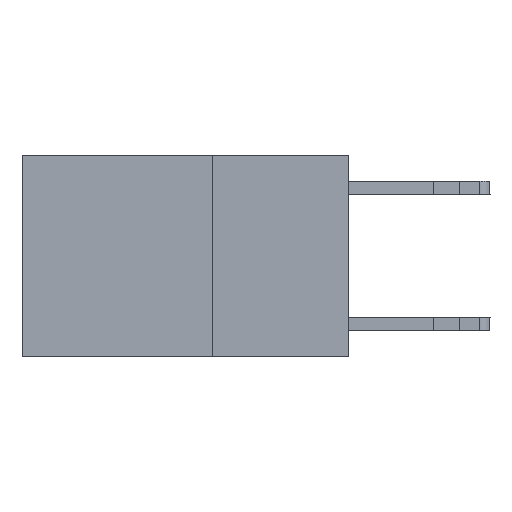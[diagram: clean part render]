
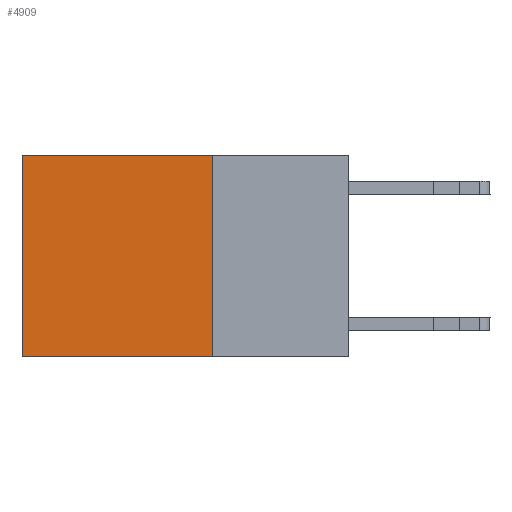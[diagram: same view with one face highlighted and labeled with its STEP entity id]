
A CAD part, left-side view. The second image highlights one B-rep face of the part: STEP entity #4909.
In plain terms, the highlighted planar face has unit normal (-1, 0, 0).
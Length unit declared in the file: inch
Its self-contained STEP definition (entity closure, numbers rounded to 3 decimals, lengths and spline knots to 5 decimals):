
#297 = CARTESIAN_POINT ( 'NONE',  ( 0.2625, 0.6, -0.37 ) ) ;
#892 = LINE ( 'NONE', #8698, #6303 ) ;
#1052 = DIRECTION ( 'NONE',  ( 0., 1., 0. ) ) ;
#1082 = FACE_OUTER_BOUND ( 'NONE', #6293, .T. ) ;
#2631 = LINE ( 'NONE', #5097, #3116 ) ;
#2633 = DIRECTION ( 'NONE',  ( 0., 0., -1. ) ) ;
#2708 = LINE ( 'NONE', #5101, #10578 ) ;
#3116 = VECTOR ( 'NONE', #7689, 39.37008 ) ;
#3671 = DIRECTION ( 'NONE',  ( 0., 1., 0. ) ) ;
#4557 = CARTESIAN_POINT ( 'NONE',  ( 0.2625, 0.25, 0. ) ) ;
#4909 = ADVANCED_FACE ( 'NONE', ( #1082 ), #15924, .F. ) ;
#5097 = CARTESIAN_POINT ( 'NONE',  ( 0.2625, 0.6, 0. ) ) ;
#5101 = CARTESIAN_POINT ( 'NONE',  ( 0.2625, 0.25, 0. ) ) ;
#5725 = ORIENTED_EDGE ( 'NONE', *, *, #12442, .F. ) ;
#5885 = DIRECTION ( 'NONE',  ( 1., 0., 0. ) ) ;
#6293 = EDGE_LOOP ( 'NONE', ( #11860, #11169, #5725, #8521 ) ) ;
#6303 = VECTOR ( 'NONE', #1052, 39.37008 ) ;
#7452 = EDGE_CURVE ( 'NONE', #13725, #13801, #892, .T. ) ;
#7689 = DIRECTION ( 'NONE',  ( 0., 0., -1. ) ) ;
#8521 = ORIENTED_EDGE ( 'NONE', *, *, #7452, .T. ) ;
#8678 = LINE ( 'NONE', #10264, #11875 ) ;
#8698 = CARTESIAN_POINT ( 'NONE',  ( 0.2625, 0.25, 0. ) ) ;
#9627 = CARTESIAN_POINT ( 'NONE',  ( 0.2625, 0.6, 0. ) ) ;
#10264 = CARTESIAN_POINT ( 'NONE',  ( 0.2625, 0.25, -0.37 ) ) ;
#10578 = VECTOR ( 'NONE', #2633, 39.37008 ) ;
#10950 = DIRECTION ( 'NONE',  ( 0., 0., -1. ) ) ;
#11169 = ORIENTED_EDGE ( 'NONE', *, *, #14357, .F. ) ;
#11860 = ORIENTED_EDGE ( 'NONE', *, *, #14031, .T. ) ;
#11875 = VECTOR ( 'NONE', #3671, 39.37008 ) ;
#12064 = AXIS2_PLACEMENT_3D ( 'NONE', #4557, #5885, #10950 ) ;
#12270 = CARTESIAN_POINT ( 'NONE',  ( 0.2625, 0.25, -0.37 ) ) ;
#12442 = EDGE_CURVE ( 'NONE', #13725, #14754, #2708, .T. ) ;
#13725 = VERTEX_POINT ( 'NONE', #14869 ) ;
#13801 = VERTEX_POINT ( 'NONE', #9627 ) ;
#14031 = EDGE_CURVE ( 'NONE', #13801, #15481, #2631, .T. ) ;
#14357 = EDGE_CURVE ( 'NONE', #14754, #15481, #8678, .T. ) ;
#14754 = VERTEX_POINT ( 'NONE', #12270 ) ;
#14869 = CARTESIAN_POINT ( 'NONE',  ( 0.2625, 0.25, 0. ) ) ;
#15481 = VERTEX_POINT ( 'NONE', #297 ) ;
#15924 = PLANE ( 'NONE',  #12064 ) ;
